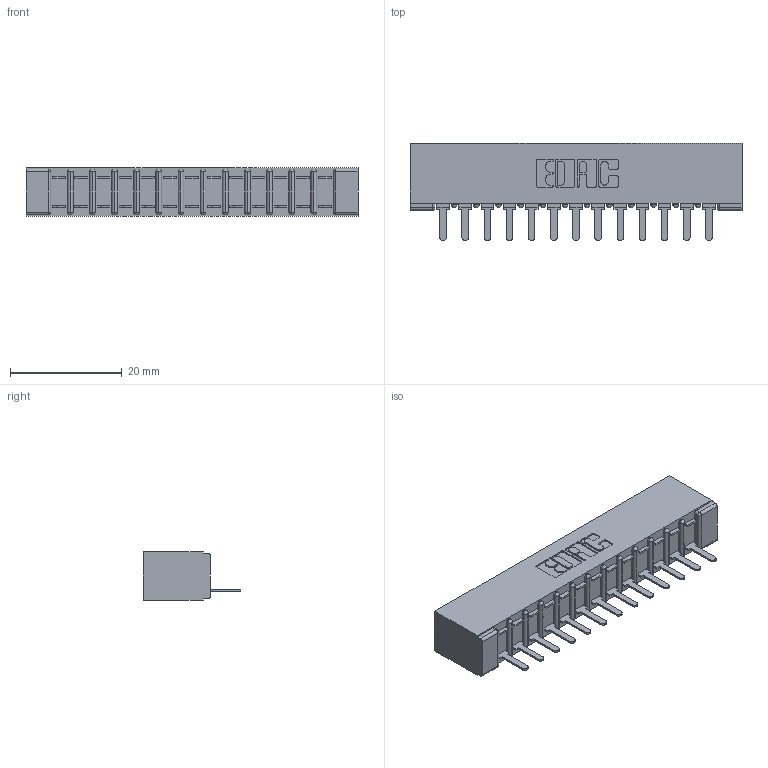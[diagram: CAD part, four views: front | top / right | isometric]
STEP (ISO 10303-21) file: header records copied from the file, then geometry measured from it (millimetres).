
FILE_DESCRIPTION (( 'STEP AP203' ), '1' );
FILE_NAME ('307-013-421-101.STEP', '2020-09-25T13:46:39', ( '' ), ( '' ), 'SwSTEP 2.0', 'SolidWorks 2020', '' );
FILE_SCHEMA (( 'CONFIG_CONTROL_DESIGN' ));
Length unit declared in the file: inch
Products named in the file (3): 307 Part_No Mounting Lugs; 307-290-002_521; 307-013-421-101
Assembly tree (14 placements, depth 2):
  307-013-421-101
    307 Part_No Mounting Lugs
    307-290-002_521  x13
Bounding box: 59.39 x 17.42 x 8.71 mm (x, y, z)
Volume: 4158.9 mm3; surface area: 7578.8 mm2
Topology: 14 solids, 14 shells, 1086 faces, 3315 edges, 2170 vertices
Faces by surface type: plane 651, cylinder 407, sphere 28
Entity records: 15160 total; most frequent: CARTESIAN_POINT 2552, ORIENTED_EDGE 2542, DIRECTION 2491, EDGE_CURVE 1271, LINE 961, VECTOR 961, VERTEX_POINT 826, AXIS2_PLACEMENT_3D 765
